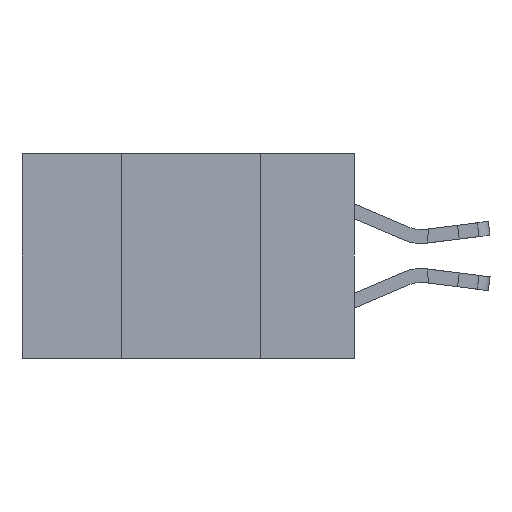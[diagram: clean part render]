
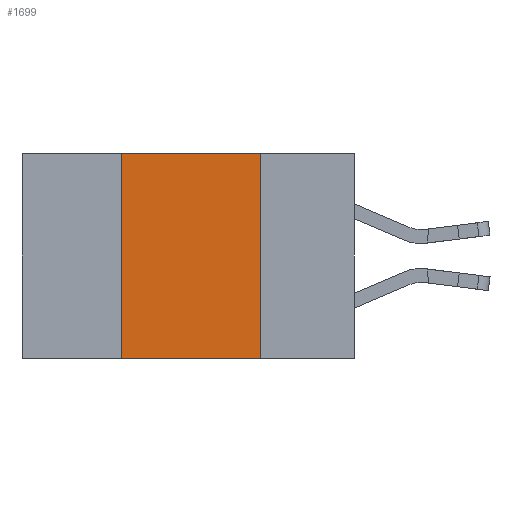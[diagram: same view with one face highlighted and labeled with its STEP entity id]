
A CAD part, left-side view. The second image highlights one B-rep face of the part: STEP entity #1699.
In plain terms, the highlighted planar face has unit normal (-1, 0, 0).
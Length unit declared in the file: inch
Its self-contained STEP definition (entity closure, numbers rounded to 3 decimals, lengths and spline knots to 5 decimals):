
#149 = ORIENTED_EDGE ( 'NONE', *, *, #10120, .T. ) ;
#253 = CARTESIAN_POINT ( 'NONE',  ( 0., 0.6, 0. ) ) ;
#940 = DIRECTION ( 'NONE',  ( 1., 0., 0. ) ) ;
#1116 = DIRECTION ( 'NONE',  ( 0., -1., 0. ) ) ;
#1699 = ADVANCED_FACE ( 'NONE', ( #4898 ), #2983, .F. ) ;
#1728 = EDGE_LOOP ( 'NONE', ( #7472, #11232, #3159, #149 ) ) ;
#2030 = EDGE_CURVE ( 'NONE', #11422, #9826, #6611, .T. ) ;
#2254 = DIRECTION ( 'NONE',  ( 0., 0., 1. ) ) ;
#2325 = VERTEX_POINT ( 'NONE', #2748 ) ;
#2547 = VECTOR ( 'NONE', #2254, 39.37008 ) ;
#2748 = CARTESIAN_POINT ( 'NONE',  ( 0., 0.17, 0. ) ) ;
#2983 = PLANE ( 'NONE',  #8587 ) ;
#3159 = ORIENTED_EDGE ( 'NONE', *, *, #2030, .F. ) ;
#3887 = CARTESIAN_POINT ( 'NONE',  ( 0., 0.17, 0. ) ) ;
#4898 = FACE_OUTER_BOUND ( 'NONE', #1728, .T. ) ;
#5509 = VECTOR ( 'NONE', #5874, 39.37008 ) ;
#5874 = DIRECTION ( 'NONE',  ( 0., 0., -1. ) ) ;
#6259 = VECTOR ( 'NONE', #1116, 39.37008 ) ;
#6611 = LINE ( 'NONE', #9202, #2547 ) ;
#6804 = DIRECTION ( 'NONE',  ( 0., -1., 0. ) ) ;
#6974 = CARTESIAN_POINT ( 'NONE',  ( 0., 0.42, 0. ) ) ;
#7197 = CARTESIAN_POINT ( 'NONE',  ( 0., 0.17, -0.37 ) ) ;
#7345 = LINE ( 'NONE', #3887, #5509 ) ;
#7472 = ORIENTED_EDGE ( 'NONE', *, *, #7734, .F. ) ;
#7734 = EDGE_CURVE ( 'NONE', #2325, #10615, #7345, .T. ) ;
#7803 = CARTESIAN_POINT ( 'NONE',  ( 0., 0.6, 0. ) ) ;
#8220 = EDGE_CURVE ( 'NONE', #9826, #2325, #11575, .T. ) ;
#8587 = AXIS2_PLACEMENT_3D ( 'NONE', #7803, #940, #8796 ) ;
#8796 = DIRECTION ( 'NONE',  ( 0., 0., -1. ) ) ;
#8823 = CARTESIAN_POINT ( 'NONE',  ( 0., 0.6, -0.37 ) ) ;
#9202 = CARTESIAN_POINT ( 'NONE',  ( 0., 0.42, 0. ) ) ;
#9826 = VERTEX_POINT ( 'NONE', #6974 ) ;
#9899 = CARTESIAN_POINT ( 'NONE',  ( 0., 0.42, -0.37 ) ) ;
#10120 = EDGE_CURVE ( 'NONE', #11422, #10615, #11930, .T. ) ;
#10615 = VERTEX_POINT ( 'NONE', #7197 ) ;
#11232 = ORIENTED_EDGE ( 'NONE', *, *, #8220, .F. ) ;
#11422 = VERTEX_POINT ( 'NONE', #9899 ) ;
#11575 = LINE ( 'NONE', #253, #6259 ) ;
#11930 = LINE ( 'NONE', #8823, #12230 ) ;
#12230 = VECTOR ( 'NONE', #6804, 39.37008 ) ;
